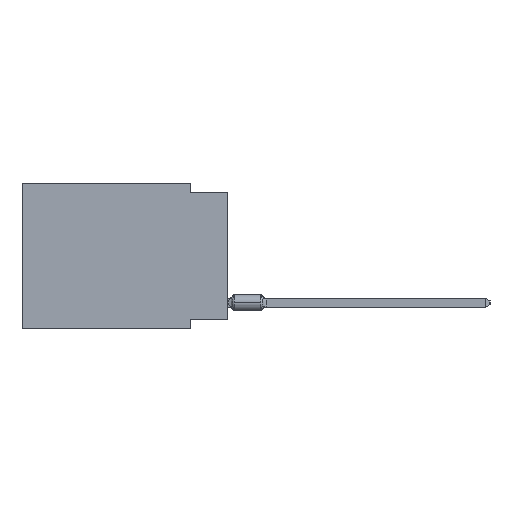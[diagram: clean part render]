
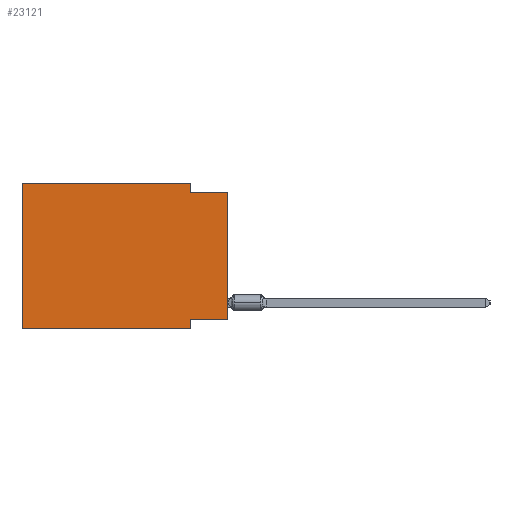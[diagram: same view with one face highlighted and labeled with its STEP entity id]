
A CAD part, left-side view. The second image highlights one B-rep face of the part: STEP entity #23121.
In plain terms, the highlighted planar face has unit normal (-1, 0, 0).
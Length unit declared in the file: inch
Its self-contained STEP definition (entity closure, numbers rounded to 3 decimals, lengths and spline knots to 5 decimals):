
#1951 = VERTEX_POINT ( 'NONE', #16425 ) ;
#2684 = DIRECTION ( 'NONE',  ( 0., -1., 0. ) ) ;
#3195 = VECTOR ( 'NONE', #19080, 39.37008 ) ;
#3886 = VECTOR ( 'NONE', #42791, 39.37008 ) ;
#3893 = VERTEX_POINT ( 'NONE', #44490 ) ;
#5531 = DIRECTION ( 'NONE',  ( 0., -1., 0. ) ) ;
#6433 = AXIS2_PLACEMENT_3D ( 'NONE', #16279, #7263, #53317 ) ;
#7263 = DIRECTION ( 'NONE',  ( 1., 0., 0. ) ) ;
#10537 = VERTEX_POINT ( 'NONE', #51696 ) ;
#12177 = FACE_OUTER_BOUND ( 'NONE', #16975, .T. ) ;
#12999 = DIRECTION ( 'NONE',  ( 0., 0., 1. ) ) ;
#13571 = VECTOR ( 'NONE', #41681, 39.37008 ) ;
#15327 = EDGE_CURVE ( 'NONE', #20311, #1951, #37695, .T. ) ;
#15594 = VERTEX_POINT ( 'NONE', #49346 ) ;
#15802 = EDGE_CURVE ( 'NONE', #10537, #32130, #21837, .T. ) ;
#16063 = ORIENTED_EDGE ( 'NONE', *, *, #21225, .F. ) ;
#16279 = CARTESIAN_POINT ( 'NONE',  ( 0., 0.55, 0. ) ) ;
#16341 = CARTESIAN_POINT ( 'NONE',  ( 0., 0.55, -0.39 ) ) ;
#16425 = CARTESIAN_POINT ( 'NONE',  ( 0., 0.55, 0. ) ) ;
#16606 = CARTESIAN_POINT ( 'NONE',  ( 0., 0.1, -0.39 ) ) ;
#16975 = EDGE_LOOP ( 'NONE', ( #34049, #50235, #27390, #16063, #21241, #40554, #22629, #32292 ) ) ;
#18964 = VERTEX_POINT ( 'NONE', #35680 ) ;
#19080 = DIRECTION ( 'NONE',  ( 0., 1., 0. ) ) ;
#19341 = LINE ( 'NONE', #27802, #3195 ) ;
#20311 = VERTEX_POINT ( 'NONE', #16341 ) ;
#20650 = CARTESIAN_POINT ( 'NONE',  ( 0., 0.1, -0.365 ) ) ;
#20767 = EDGE_CURVE ( 'NONE', #3893, #18964, #50327, .T. ) ;
#21225 = EDGE_CURVE ( 'NONE', #1951, #10537, #26266, .T. ) ;
#21241 = ORIENTED_EDGE ( 'NONE', *, *, #15327, .F. ) ;
#21837 = LINE ( 'NONE', #34336, #3886 ) ;
#21892 = CARTESIAN_POINT ( 'NONE',  ( 0., 0.55, 0. ) ) ;
#22629 = ORIENTED_EDGE ( 'NONE', *, *, #28616, .F. ) ;
#23121 = ADVANCED_FACE ( 'NONE', ( #12177 ), #48695, .F. ) ;
#24432 = CARTESIAN_POINT ( 'NONE',  ( 0., 0., 0. ) ) ;
#25972 = DIRECTION ( 'NONE',  ( 0., 0., 1. ) ) ;
#26266 = LINE ( 'NONE', #42870, #30698 ) ;
#27390 = ORIENTED_EDGE ( 'NONE', *, *, #15802, .F. ) ;
#27802 = CARTESIAN_POINT ( 'NONE',  ( 0., 0., -0.365 ) ) ;
#28616 = EDGE_CURVE ( 'NONE', #43291, #15594, #50113, .T. ) ;
#29806 = VECTOR ( 'NONE', #12999, 39.37008 ) ;
#30698 = VECTOR ( 'NONE', #5531, 39.37008 ) ;
#30793 = LINE ( 'NONE', #48208, #51790 ) ;
#31917 = CARTESIAN_POINT ( 'NONE',  ( 0., 0.1, -0.025 ) ) ;
#32130 = VERTEX_POINT ( 'NONE', #31917 ) ;
#32292 = ORIENTED_EDGE ( 'NONE', *, *, #41993, .F. ) ;
#34049 = ORIENTED_EDGE ( 'NONE', *, *, #20767, .T. ) ;
#34336 = CARTESIAN_POINT ( 'NONE',  ( 0., 0.1, 0. ) ) ;
#35680 = CARTESIAN_POINT ( 'NONE',  ( 0., 0., -0.025 ) ) ;
#36179 = EDGE_CURVE ( 'NONE', #20311, #15594, #30793, .T. ) ;
#37695 = LINE ( 'NONE', #21892, #42296 ) ;
#40554 = ORIENTED_EDGE ( 'NONE', *, *, #36179, .T. ) ;
#41681 = DIRECTION ( 'NONE',  ( 0., -1., 0. ) ) ;
#41993 = EDGE_CURVE ( 'NONE', #3893, #43291, #19341, .T. ) ;
#42296 = VECTOR ( 'NONE', #25972, 39.37008 ) ;
#42791 = DIRECTION ( 'NONE',  ( 0., 0., -1. ) ) ;
#42870 = CARTESIAN_POINT ( 'NONE',  ( 0., 0.55, 0. ) ) ;
#43291 = VERTEX_POINT ( 'NONE', #20650 ) ;
#44380 = DIRECTION ( 'NONE',  ( 0., 0., -1. ) ) ;
#44490 = CARTESIAN_POINT ( 'NONE',  ( 0., 0., -0.365 ) ) ;
#46320 = LINE ( 'NONE', #49870, #13571 ) ;
#48208 = CARTESIAN_POINT ( 'NONE',  ( 0., 0.55, -0.39 ) ) ;
#48695 = PLANE ( 'NONE',  #6433 ) ;
#48803 = EDGE_CURVE ( 'NONE', #32130, #18964, #46320, .T. ) ;
#49346 = CARTESIAN_POINT ( 'NONE',  ( 0., 0.1, -0.39 ) ) ;
#49379 = VECTOR ( 'NONE', #44380, 39.37008 ) ;
#49870 = CARTESIAN_POINT ( 'NONE',  ( 0., 0., -0.025 ) ) ;
#50113 = LINE ( 'NONE', #16606, #49379 ) ;
#50235 = ORIENTED_EDGE ( 'NONE', *, *, #48803, .F. ) ;
#50327 = LINE ( 'NONE', #24432, #29806 ) ;
#51696 = CARTESIAN_POINT ( 'NONE',  ( 0., 0.1, 0. ) ) ;
#51790 = VECTOR ( 'NONE', #2684, 39.37008 ) ;
#53317 = DIRECTION ( 'NONE',  ( 0., 0., -1. ) ) ;
